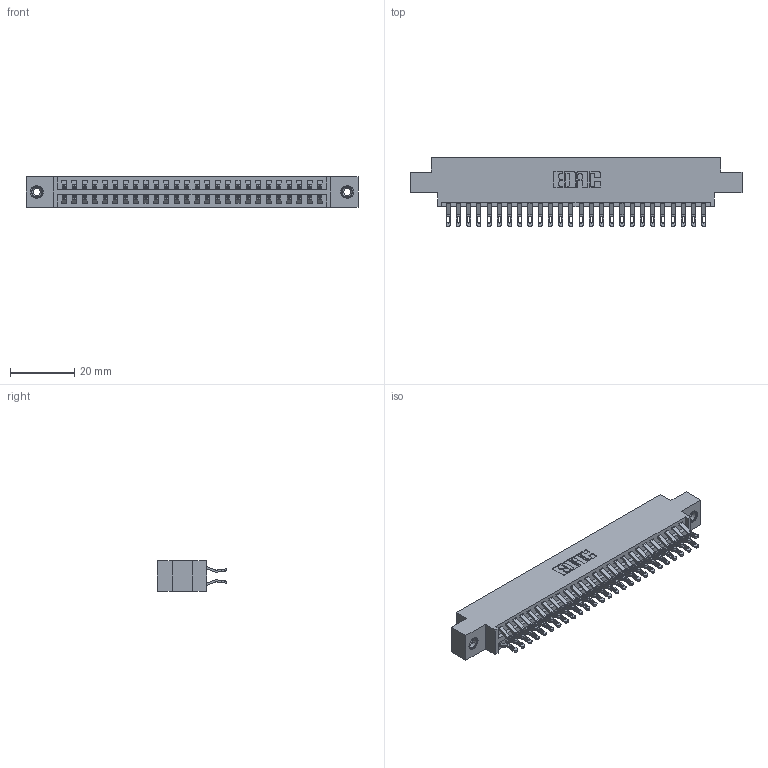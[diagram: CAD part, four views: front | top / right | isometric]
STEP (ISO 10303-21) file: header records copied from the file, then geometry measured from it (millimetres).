
FILE_DESCRIPTION (( 'STEP AP203' ), '1' );
FILE_NAME ('346-052-555-808.STEP', '2022-05-21T01:41:14', ( '' ), ( '' ), 'SwSTEP 2.0', 'SolidWorks 2020', '' );
FILE_SCHEMA (( 'CONFIG_CONTROL_DESIGN' ));
Length unit declared in the file: inch
Products named in the file (4): 346 Part_0.170 Offset - 0.156 Dia-TI; 345-250-001_345-250-003-102; 345-292-001_555 Tail; 346-052-555-808
Assembly tree (55 placements, depth 2):
  346-052-555-808
    346 Part_0.170 Offset - 0.156 Dia-TI
    345-292-001_555 Tail  x52
    345-250-001_345-250-003-102  x2
Bounding box: 103.12 x 21.46 x 9.4 mm (x, y, z)
Volume: 9921.3 mm3; surface area: 14123.3 mm2
Topology: 55 solids, 55 shells, 3202 faces, 9993 edges, 6654 vertices
Faces by surface type: plane 1828, cylinder 1358, cone 12, torus 4
Entity records: 20766 total; most frequent: CARTESIAN_POINT 3465, ORIENTED_EDGE 3362, DIRECTION 3099, EDGE_CURVE 1681, VECTOR 1405, LINE 1405, VERTEX_POINT 1116, AXIS2_PLACEMENT_3D 847
